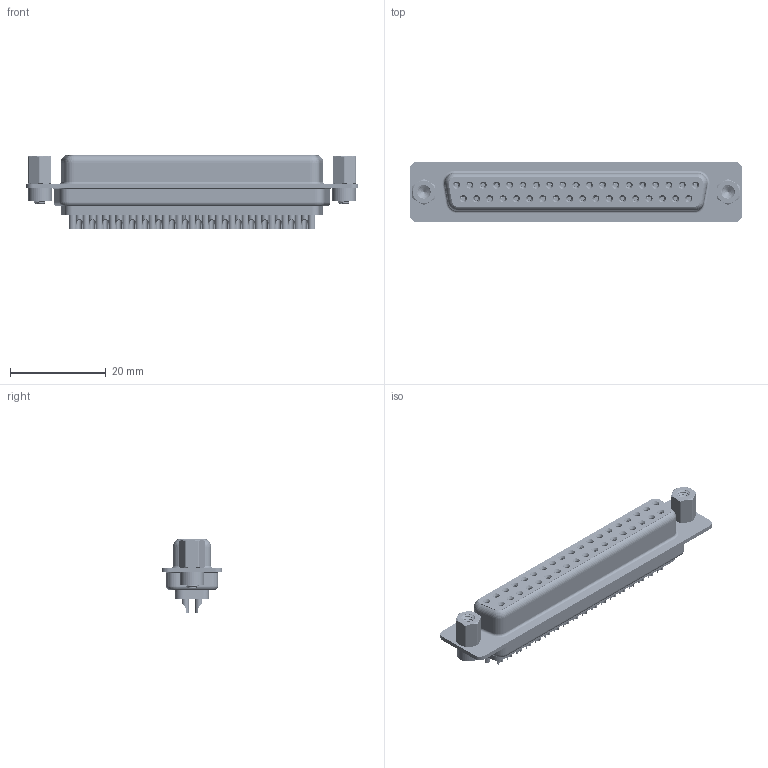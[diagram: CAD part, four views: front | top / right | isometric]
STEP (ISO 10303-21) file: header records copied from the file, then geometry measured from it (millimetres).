
FILE_DESCRIPTION (( 'STEP AP203' ), '1' );
FILE_NAME ('628-037-622-543.STEP', '2018-10-20T05:21:23', ( '' ), ( '' ), 'SwSTEP 2.0', 'SolidWorks 2016', '' );
FILE_SCHEMA (( 'CONFIG_CONTROL_DESIGN' ));
Length unit declared in the file: millimetre
Products named in the file (8): 628 Contact Row 2_22L; 628 4-40 Threaded Rivet; 628 4-40 Hex Standoff; 628-037-622-543; 628 Housing_37 LP; 628 Shell Front_37 Contacts; 628 Shell Rear_37 Contacts; 628 Contact Row 1_22L
Assembly tree (44 placements, depth 2):
  628-037-622-543
    628 Housing_37 LP
    628 Shell Front_37 Contacts
    628 Shell Rear_37 Contacts
    628 Contact Row 1_22L  x19
    628 Contact Row 2_22L  x18
    628 4-40 Threaded Rivet  x2
    628 4-40 Hex Standoff  x2
Bounding box: 69.3 x 12.6 x 15.35 mm (x, y, z)
Volume: 6031.4 mm3; surface area: 14167.1 mm2
Topology: 44 solids, 44 shells, 3671 faces, 9330 edges, 5870 vertices
Faces by surface type: cylinder 1121, plane 863, bspline 758, torus 718, cone 211
Entity records: 34137 total; most frequent: CARTESIAN_POINT 10895, DIRECTION 4737, ORIENTED_EDGE 4284, EDGE_CURVE 2142, AXIS2_PLACEMENT_3D 1991, VERTEX_POINT 1364, EDGE_LOOP 1124, CIRCLE 1078
